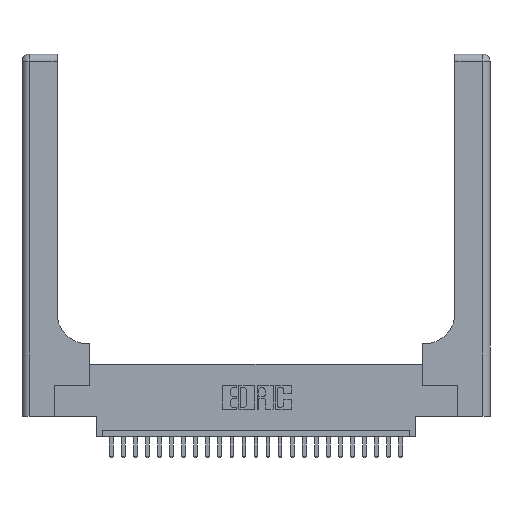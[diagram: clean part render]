
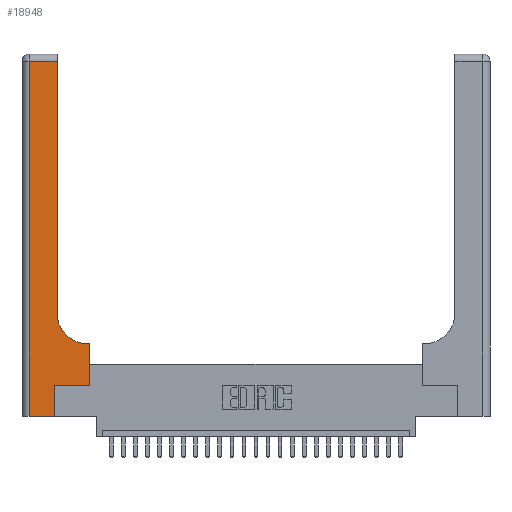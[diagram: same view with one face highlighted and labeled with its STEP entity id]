
A CAD part, top view. The second image highlights one B-rep face of the part: STEP entity #18948.
In plain terms, the highlighted planar face has unit normal (0, 0, 1).
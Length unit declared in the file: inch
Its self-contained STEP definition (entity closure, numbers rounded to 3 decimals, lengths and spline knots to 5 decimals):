
#166 = DIRECTION ( 'NONE',  ( 0., 1., 0. ) ) ;
#510 = VECTOR ( 'NONE', #22017, 39.37008 ) ;
#841 = LINE ( 'NONE', #3090, #510 ) ;
#1529 = CARTESIAN_POINT ( 'NONE',  ( 0., 2.94, 0.37 ) ) ;
#1930 = LINE ( 'NONE', #18439, #16689 ) ;
#1989 = CARTESIAN_POINT ( 'NONE',  ( 0.269, 0., 0.37 ) ) ;
#2685 = EDGE_LOOP ( 'NONE', ( #15518, #3789, #15543, #15137, #23019, #24493, #3673, #22449, #15579 ) ) ;
#3072 = CARTESIAN_POINT ( 'NONE',  ( 0.2915, 0.85, 0.37 ) ) ;
#3090 = CARTESIAN_POINT ( 'NONE',  ( 0.06, 3., 0.37 ) ) ;
#3460 = DIRECTION ( 'NONE',  ( 0., 1., 0. ) ) ;
#3673 = ORIENTED_EDGE ( 'NONE', *, *, #16128, .T. ) ;
#3789 = ORIENTED_EDGE ( 'NONE', *, *, #5545, .T. ) ;
#3970 = LINE ( 'NONE', #9906, #14238 ) ;
#4817 = VERTEX_POINT ( 'NONE', #21858 ) ;
#5505 = VERTEX_POINT ( 'NONE', #3072 ) ;
#5545 = EDGE_CURVE ( 'NONE', #12893, #25680, #23894, .T. ) ;
#5622 = CARTESIAN_POINT ( 'NONE',  ( 0.269, 0.25, 0.37 ) ) ;
#5797 = LINE ( 'NONE', #1989, #25307 ) ;
#6440 = CARTESIAN_POINT ( 'NONE',  ( 0.2915, 0.6, 0.37 ) ) ;
#7648 = LINE ( 'NONE', #6440, #13693 ) ;
#7933 = DIRECTION ( 'NONE',  ( -1., 0., 0. ) ) ;
#8069 = LINE ( 'NONE', #11189, #25951 ) ;
#9061 = VERTEX_POINT ( 'NONE', #25556 ) ;
#9906 = CARTESIAN_POINT ( 'NONE',  ( 0.2915, 3., 0.37 ) ) ;
#10021 = DIRECTION ( 'NONE',  ( 1., 0., 0. ) ) ;
#10107 = EDGE_CURVE ( 'NONE', #4817, #21679, #10382, .T. ) ;
#10382 = LINE ( 'NONE', #24829, #15504 ) ;
#10436 = CIRCLE ( 'NONE', #23461, 0.25 ) ;
#10697 = DIRECTION ( 'NONE',  ( -1., 0., 0. ) ) ;
#11189 = CARTESIAN_POINT ( 'NONE',  ( 0.269, 0.25, 0.37 ) ) ;
#11640 = CARTESIAN_POINT ( 'NONE',  ( 0.5415, 0.85, 0.37 ) ) ;
#11996 = DIRECTION ( 'NONE',  ( 1., 0., 0. ) ) ;
#12200 = EDGE_CURVE ( 'NONE', #20457, #23323, #8069, .T. ) ;
#12602 = DIRECTION ( 'NONE',  ( 1., 0., 0. ) ) ;
#12893 = VERTEX_POINT ( 'NONE', #16555 ) ;
#13693 = VECTOR ( 'NONE', #10697, 39.37008 ) ;
#13746 = CARTESIAN_POINT ( 'NONE',  ( 0., 3., 0.37 ) ) ;
#13921 = DIRECTION ( 'NONE',  ( -1., 0., 0. ) ) ;
#14238 = VECTOR ( 'NONE', #3460, 39.37008 ) ;
#14933 = EDGE_CURVE ( 'NONE', #21159, #9061, #7648, .T. ) ;
#15137 = ORIENTED_EDGE ( 'NONE', *, *, #10107, .T. ) ;
#15145 = EDGE_CURVE ( 'NONE', #25680, #4817, #841, .T. ) ;
#15504 = VECTOR ( 'NONE', #12602, 39.37008 ) ;
#15518 = ORIENTED_EDGE ( 'NONE', *, *, #20448, .T. ) ;
#15543 = ORIENTED_EDGE ( 'NONE', *, *, #15145, .T. ) ;
#15579 = ORIENTED_EDGE ( 'NONE', *, *, #24280, .T. ) ;
#15707 = CARTESIAN_POINT ( 'NONE',  ( 0.5585, 0.25, 0.37 ) ) ;
#15810 = DIRECTION ( 'NONE',  ( 0., 0., -1. ) ) ;
#16128 = EDGE_CURVE ( 'NONE', #23323, #21159, #1930, .T. ) ;
#16187 = EDGE_CURVE ( 'NONE', #21679, #20457, #5797, .T. ) ;
#16433 = DIRECTION ( 'NONE',  ( 0., 1., 0. ) ) ;
#16555 = CARTESIAN_POINT ( 'NONE',  ( 0.2915, 2.94, 0.37 ) ) ;
#16689 = VECTOR ( 'NONE', #16433, 39.37008 ) ;
#16844 = AXIS2_PLACEMENT_3D ( 'NONE', #13746, #15810, #13921 ) ;
#17086 = CARTESIAN_POINT ( 'NONE',  ( 0.269, 0., 0.37 ) ) ;
#17651 = PLANE ( 'NONE',  #16844 ) ;
#18439 = CARTESIAN_POINT ( 'NONE',  ( 0.5585, 0.25, 0.37 ) ) ;
#18948 = ADVANCED_FACE ( 'NONE', ( #26151 ), #17651, .F. ) ;
#19870 = CARTESIAN_POINT ( 'NONE',  ( 0.06, 2.94, 0.37 ) ) ;
#20448 = EDGE_CURVE ( 'NONE', #5505, #12893, #3970, .T. ) ;
#20457 = VERTEX_POINT ( 'NONE', #5622 ) ;
#21159 = VERTEX_POINT ( 'NONE', #25656 ) ;
#21679 = VERTEX_POINT ( 'NONE', #17086 ) ;
#21858 = CARTESIAN_POINT ( 'NONE',  ( 0.06, 0., 0.37 ) ) ;
#22017 = DIRECTION ( 'NONE',  ( 0., -1., 0. ) ) ;
#22449 = ORIENTED_EDGE ( 'NONE', *, *, #14933, .T. ) ;
#22929 = VECTOR ( 'NONE', #7933, 39.37008 ) ;
#23019 = ORIENTED_EDGE ( 'NONE', *, *, #16187, .T. ) ;
#23323 = VERTEX_POINT ( 'NONE', #15707 ) ;
#23461 = AXIS2_PLACEMENT_3D ( 'NONE', #11640, #25945, #11996 ) ;
#23894 = LINE ( 'NONE', #1529, #22929 ) ;
#24280 = EDGE_CURVE ( 'NONE', #9061, #5505, #10436, .T. ) ;
#24493 = ORIENTED_EDGE ( 'NONE', *, *, #12200, .T. ) ;
#24829 = CARTESIAN_POINT ( 'NONE',  ( 0., 0., 0.37 ) ) ;
#25307 = VECTOR ( 'NONE', #166, 39.37008 ) ;
#25556 = CARTESIAN_POINT ( 'NONE',  ( 0.5415, 0.6, 0.37 ) ) ;
#25656 = CARTESIAN_POINT ( 'NONE',  ( 0.5585, 0.6, 0.37 ) ) ;
#25680 = VERTEX_POINT ( 'NONE', #19870 ) ;
#25945 = DIRECTION ( 'NONE',  ( 0., 0., -1. ) ) ;
#25951 = VECTOR ( 'NONE', #10021, 39.37008 ) ;
#26151 = FACE_OUTER_BOUND ( 'NONE', #2685, .T. ) ;
